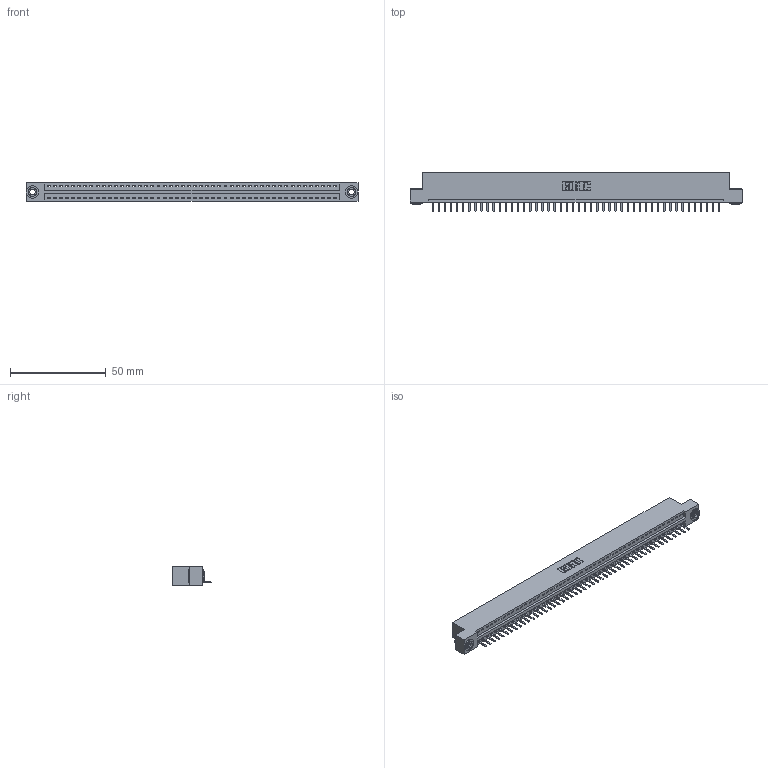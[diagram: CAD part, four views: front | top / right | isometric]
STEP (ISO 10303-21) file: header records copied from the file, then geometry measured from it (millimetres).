
FILE_DESCRIPTION (( 'STEP AP203' ), '1' );
FILE_NAME ('346-048-520-103.STEP', '2022-05-09T22:53:34', ( '' ), ( '' ), 'SwSTEP 2.0', 'SolidWorks 2020', '' );
FILE_SCHEMA (( 'CONFIG_CONTROL_DESIGN' ));
Length unit declared in the file: inch
Products named in the file (4): 346 Part_Flush Mounting Lugs - 0.156 Dia-TH; 346-048-520-103; 345-292-001_345-293-120; 345-250-002_345-250-002-102
Assembly tree (51 placements, depth 2):
  346-048-520-103
    346 Part_Flush Mounting Lugs - 0.156 Dia-TH
    345-292-001_345-293-120  x48
    345-250-002_345-250-002-102  x2
Bounding box: 172.97 x 20.02 x 9.4 mm (x, y, z)
Volume: 16462 mm3; surface area: 20430.7 mm2
Topology: 51 solids, 51 shells, 3150 faces, 9273 edges, 6050 vertices
Faces by surface type: plane 2116, cylinder 1026, cone 8
Entity records: 30162 total; most frequent: CARTESIAN_POINT 5161, ORIENTED_EDGE 5122, DIRECTION 4563, EDGE_CURVE 2561, VECTOR 2209, LINE 2209, VERTEX_POINT 1702, AXIS2_PLACEMENT_3D 1177
